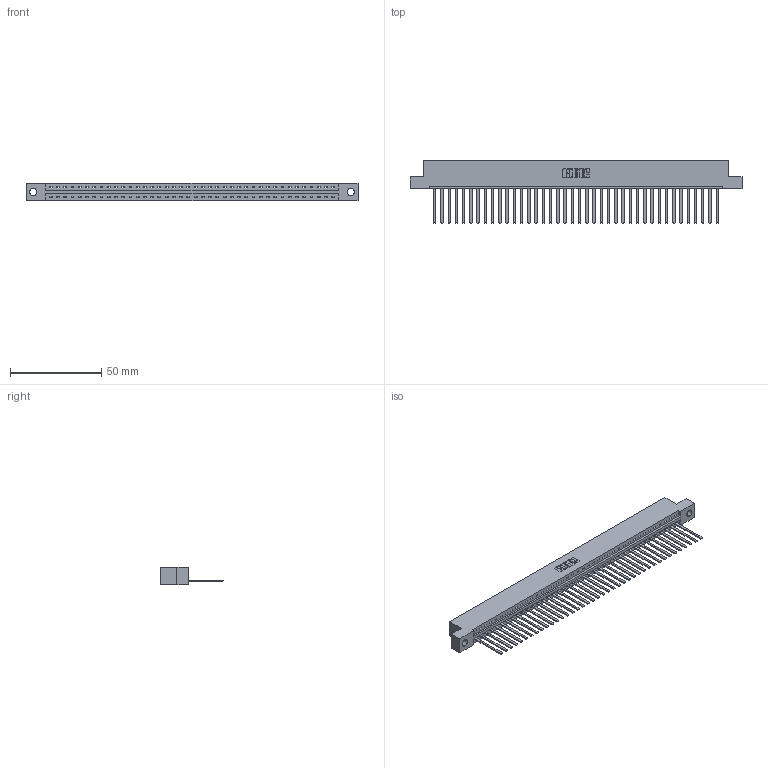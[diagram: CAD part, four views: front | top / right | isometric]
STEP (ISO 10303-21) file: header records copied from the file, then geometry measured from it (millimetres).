
FILE_DESCRIPTION (( 'STEP AP203' ), '1' );
FILE_NAME ('387-040-544-104.STEP', '2018-09-19T16:36:49', ( '' ), ( '' ), 'SwSTEP 2.0', 'SolidWorks 2016', '' );
FILE_SCHEMA (( 'CONFIG_CONTROL_DESIGN' ));
Length unit declared in the file: inch
Products named in the file (3): 387-040-544-104; 337 Part_Flush Mounting Lugs - 0.156 Dia-TH; 345-292-001_345-293-144
Assembly tree (41 placements, depth 2):
  387-040-544-104
    337 Part_Flush Mounting Lugs - 0.156 Dia-TH
    345-292-001_345-293-144  x40
Bounding box: 181.51 x 34.3 x 9.4 mm (x, y, z)
Volume: 19215.1 mm3; surface area: 21164.1 mm2
Topology: 41 solids, 41 shells, 2354 faces, 7111 edges, 4686 vertices
Faces by surface type: plane 1750, cylinder 604
Entity records: 29811 total; most frequent: CARTESIAN_POINT 5198, ORIENTED_EDGE 5174, DIRECTION 4375, EDGE_CURVE 2587, VECTOR 2463, LINE 2463, VERTEX_POINT 1722, AXIS2_PLACEMENT_3D 956
